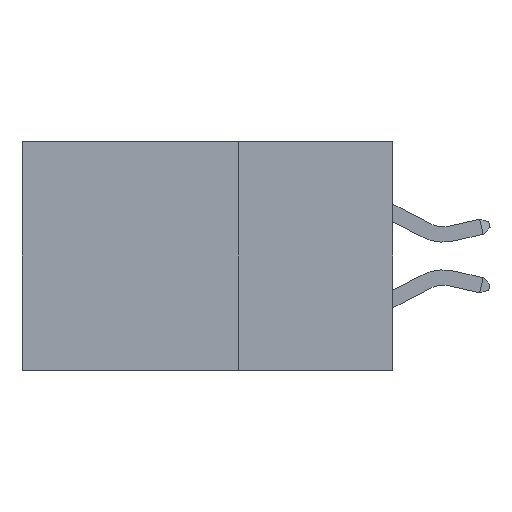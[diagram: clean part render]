
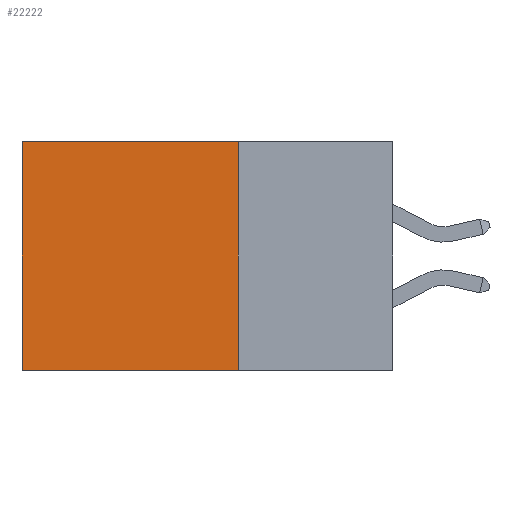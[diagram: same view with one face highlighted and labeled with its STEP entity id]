
A CAD part, left-side view. The second image highlights one B-rep face of the part: STEP entity #22222.
In plain terms, the highlighted planar face has unit normal (-1, 0, 0).
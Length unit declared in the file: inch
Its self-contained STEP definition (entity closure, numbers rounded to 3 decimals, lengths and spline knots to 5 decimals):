
#1028 = EDGE_CURVE ( 'NONE', #2379, #15914, #14000, .T. ) ;
#1537 = CARTESIAN_POINT ( 'NONE',  ( 0.2875, 0.6, -0.37 ) ) ;
#2058 = DIRECTION ( 'NONE',  ( 0., 1., 0. ) ) ;
#2067 = ORIENTED_EDGE ( 'NONE', *, *, #13576, .F. ) ;
#2379 = VERTEX_POINT ( 'NONE', #14830 ) ;
#3940 = CARTESIAN_POINT ( 'NONE',  ( 0.2875, 0.6, 0. ) ) ;
#4077 = CARTESIAN_POINT ( 'NONE',  ( 0.2875, 0.6, 0. ) ) ;
#5336 = LINE ( 'NONE', #3940, #21826 ) ;
#5451 = CARTESIAN_POINT ( 'NONE',  ( 0.2875, 0.25, 0. ) ) ;
#7953 = CARTESIAN_POINT ( 'NONE',  ( 0.2875, 0.25, 0. ) ) ;
#8234 = VECTOR ( 'NONE', #22407, 39.37008 ) ;
#9171 = CARTESIAN_POINT ( 'NONE',  ( 0.2875, 0.25, 0. ) ) ;
#9227 = DIRECTION ( 'NONE',  ( 0., 0., -1. ) ) ;
#9549 = EDGE_LOOP ( 'NONE', ( #19300, #19636, #2067, #13066 ) ) ;
#9714 = LINE ( 'NONE', #22755, #8234 ) ;
#11256 = EDGE_CURVE ( 'NONE', #16455, #13403, #18042, .T. ) ;
#12898 = DIRECTION ( 'NONE',  ( 0., 1., 0. ) ) ;
#13066 = ORIENTED_EDGE ( 'NONE', *, *, #11256, .T. ) ;
#13403 = VERTEX_POINT ( 'NONE', #4077 ) ;
#13576 = EDGE_CURVE ( 'NONE', #16455, #2379, #9714, .T. ) ;
#14000 = LINE ( 'NONE', #21830, #21003 ) ;
#14830 = CARTESIAN_POINT ( 'NONE',  ( 0.2875, 0.25, -0.37 ) ) ;
#15914 = VERTEX_POINT ( 'NONE', #1537 ) ;
#16333 = DIRECTION ( 'NONE',  ( 0., 0., -1. ) ) ;
#16455 = VERTEX_POINT ( 'NONE', #7953 ) ;
#17646 = AXIS2_PLACEMENT_3D ( 'NONE', #9171, #19975, #16333 ) ;
#18042 = LINE ( 'NONE', #5451, #20795 ) ;
#19300 = ORIENTED_EDGE ( 'NONE', *, *, #23154, .T. ) ;
#19636 = ORIENTED_EDGE ( 'NONE', *, *, #1028, .F. ) ;
#19975 = DIRECTION ( 'NONE',  ( 1., 0., 0. ) ) ;
#20200 = PLANE ( 'NONE',  #17646 ) ;
#20795 = VECTOR ( 'NONE', #2058, 39.37008 ) ;
#21003 = VECTOR ( 'NONE', #12898, 39.37008 ) ;
#21826 = VECTOR ( 'NONE', #9227, 39.37008 ) ;
#21830 = CARTESIAN_POINT ( 'NONE',  ( 0.2875, 0.25, -0.37 ) ) ;
#21853 = FACE_OUTER_BOUND ( 'NONE', #9549, .T. ) ;
#22222 = ADVANCED_FACE ( 'NONE', ( #21853 ), #20200, .F. ) ;
#22407 = DIRECTION ( 'NONE',  ( 0., 0., -1. ) ) ;
#22755 = CARTESIAN_POINT ( 'NONE',  ( 0.2875, 0.25, 0. ) ) ;
#23154 = EDGE_CURVE ( 'NONE', #13403, #15914, #5336, .T. ) ;
